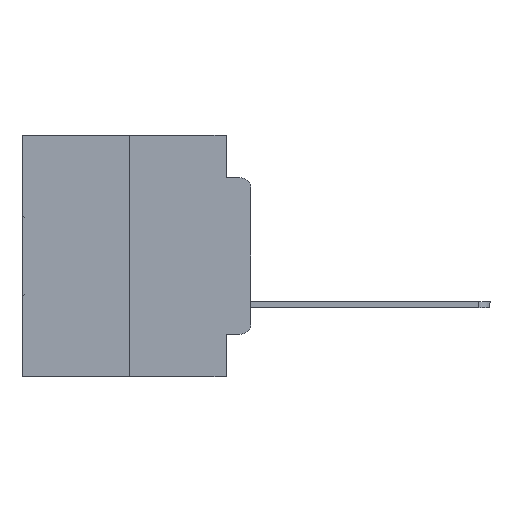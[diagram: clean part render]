
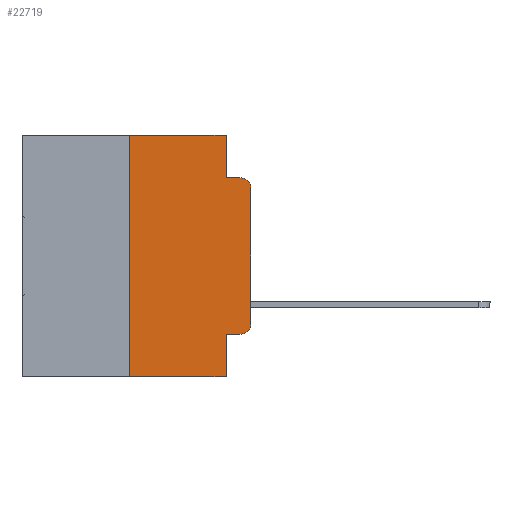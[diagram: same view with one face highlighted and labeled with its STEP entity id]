
A CAD part, left-side view. The second image highlights one B-rep face of the part: STEP entity #22719.
In plain terms, the highlighted planar face has unit normal (-1, 0, 0).
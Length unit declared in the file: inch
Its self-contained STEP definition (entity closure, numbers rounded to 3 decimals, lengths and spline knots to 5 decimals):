
#264 = DIRECTION ( 'NONE',  ( 0., -1., 0. ) ) ;
#451 = EDGE_CURVE ( 'NONE', #6566, #6896, #15571, .T. ) ;
#666 = VERTEX_POINT ( 'NONE', #14685 ) ;
#724 = EDGE_CURVE ( 'NONE', #666, #9016, #13957, .T. ) ;
#1267 = ORIENTED_EDGE ( 'NONE', *, *, #21734, .F. ) ;
#2016 = EDGE_CURVE ( 'NONE', #6903, #4729, #30139, .T. ) ;
#2399 = CARTESIAN_POINT ( 'NONE',  ( 0., 0.051, -0.4115 ) ) ;
#2629 = CARTESIAN_POINT ( 'NONE',  ( 0., 0.051, -0.0885 ) ) ;
#4120 = VECTOR ( 'NONE', #4878, 39.37008 ) ;
#4317 = ORIENTED_EDGE ( 'NONE', *, *, #24093, .F. ) ;
#4729 = VERTEX_POINT ( 'NONE', #5276 ) ;
#4870 = CARTESIAN_POINT ( 'NONE',  ( 0., 0.051, -0.0885 ) ) ;
#4878 = DIRECTION ( 'NONE',  ( 0., 0., 1. ) ) ;
#5249 = AXIS2_PLACEMENT_3D ( 'NONE', #32288, #24366, #12070 ) ;
#5276 = CARTESIAN_POINT ( 'NONE',  ( 0., 0.051, -0.5 ) ) ;
#5303 = ORIENTED_EDGE ( 'NONE', *, *, #2016, .F. ) ;
#6208 = CARTESIAN_POINT ( 'NONE',  ( 0., 0.051, 0. ) ) ;
#6566 = VERTEX_POINT ( 'NONE', #25205 ) ;
#6845 = CIRCLE ( 'NONE', #5249, 0.02 ) ;
#6870 = EDGE_CURVE ( 'NONE', #9016, #17054, #7037, .T. ) ;
#6896 = VERTEX_POINT ( 'NONE', #24810 ) ;
#6903 = VERTEX_POINT ( 'NONE', #29926 ) ;
#7037 = LINE ( 'NONE', #27613, #4120 ) ;
#7404 = DIRECTION ( 'NONE',  ( 0., 0., -1. ) ) ;
#8459 = EDGE_CURVE ( 'NONE', #6903, #666, #19506, .T. ) ;
#8486 = VECTOR ( 'NONE', #30103, 39.37008 ) ;
#9016 = VERTEX_POINT ( 'NONE', #17966 ) ;
#9528 = CARTESIAN_POINT ( 'NONE',  ( 0., 0.02, -0.3915 ) ) ;
#9905 = ORIENTED_EDGE ( 'NONE', *, *, #724, .T. ) ;
#10601 = CARTESIAN_POINT ( 'NONE',  ( 0., 0.25, 0. ) ) ;
#11735 = DIRECTION ( 'NONE',  ( 0., 0., -1. ) ) ;
#12070 = DIRECTION ( 'NONE',  ( 0., 0., -1. ) ) ;
#12193 = DIRECTION ( 'NONE',  ( -1., 0., 0. ) ) ;
#12266 = DIRECTION ( 'NONE',  ( 0., -1., 0. ) ) ;
#12525 = VECTOR ( 'NONE', #12266, 39.37008 ) ;
#12595 = CARTESIAN_POINT ( 'NONE',  ( 0., 0., -0.1085 ) ) ;
#13957 = CIRCLE ( 'NONE', #17136, 0.02 ) ;
#14685 = CARTESIAN_POINT ( 'NONE',  ( 0., 0.02, -0.4115 ) ) ;
#15571 = LINE ( 'NONE', #10601, #27659 ) ;
#15841 = DIRECTION ( 'NONE',  ( 0., -1., 0. ) ) ;
#16435 = VERTEX_POINT ( 'NONE', #28779 ) ;
#17054 = VERTEX_POINT ( 'NONE', #12595 ) ;
#17136 = AXIS2_PLACEMENT_3D ( 'NONE', #9528, #12193, #22322 ) ;
#17444 = ORIENTED_EDGE ( 'NONE', *, *, #6870, .T. ) ;
#17519 = EDGE_CURVE ( 'NONE', #6896, #16435, #20186, .T. ) ;
#17909 = DIRECTION ( 'NONE',  ( 0., 0., 1. ) ) ;
#17966 = CARTESIAN_POINT ( 'NONE',  ( 0., 0., -0.3915 ) ) ;
#18014 = CARTESIAN_POINT ( 'NONE',  ( 0., 0.473, -0.5 ) ) ;
#18182 = CARTESIAN_POINT ( 'NONE',  ( 0., 0.02, -0.0885 ) ) ;
#18297 = AXIS2_PLACEMENT_3D ( 'NONE', #24506, #29794, #7404 ) ;
#18339 = LINE ( 'NONE', #18014, #28554 ) ;
#18352 = DIRECTION ( 'NONE',  ( 0., 0., -1. ) ) ;
#18648 = EDGE_CURVE ( 'NONE', #17054, #21561, #6845, .T. ) ;
#18996 = LINE ( 'NONE', #6208, #30937 ) ;
#19506 = LINE ( 'NONE', #2399, #8486 ) ;
#19689 = FACE_OUTER_BOUND ( 'NONE', #26710, .T. ) ;
#19736 = LINE ( 'NONE', #2629, #12525 ) ;
#20086 = VECTOR ( 'NONE', #11735, 39.37008 ) ;
#20186 = LINE ( 'NONE', #29801, #31661 ) ;
#21536 = ORIENTED_EDGE ( 'NONE', *, *, #28408, .T. ) ;
#21561 = VERTEX_POINT ( 'NONE', #18182 ) ;
#21734 = EDGE_CURVE ( 'NONE', #16435, #22006, #18996, .T. ) ;
#22006 = VERTEX_POINT ( 'NONE', #4870 ) ;
#22322 = DIRECTION ( 'NONE',  ( 0., 0., -1. ) ) ;
#22719 = ADVANCED_FACE ( 'NONE', ( #19689 ), #32107, .F. ) ;
#24093 = EDGE_CURVE ( 'NONE', #22006, #21561, #19736, .T. ) ;
#24267 = ORIENTED_EDGE ( 'NONE', *, *, #18648, .T. ) ;
#24366 = DIRECTION ( 'NONE',  ( -1., 0., 0. ) ) ;
#24506 = CARTESIAN_POINT ( 'NONE',  ( 0., 0.473, 0. ) ) ;
#24518 = CARTESIAN_POINT ( 'NONE',  ( 0., 0.051, 0. ) ) ;
#24810 = CARTESIAN_POINT ( 'NONE',  ( 0., 0.25, 0. ) ) ;
#25205 = CARTESIAN_POINT ( 'NONE',  ( 0., 0.25, -0.5 ) ) ;
#26658 = ORIENTED_EDGE ( 'NONE', *, *, #451, .F. ) ;
#26710 = EDGE_LOOP ( 'NONE', ( #17444, #24267, #4317, #1267, #32604, #26658, #21536, #5303, #30514, #9905 ) ) ;
#27613 = CARTESIAN_POINT ( 'NONE',  ( 0., 0., 0. ) ) ;
#27659 = VECTOR ( 'NONE', #17909, 39.37008 ) ;
#28408 = EDGE_CURVE ( 'NONE', #6566, #4729, #18339, .T. ) ;
#28554 = VECTOR ( 'NONE', #15841, 39.37008 ) ;
#28779 = CARTESIAN_POINT ( 'NONE',  ( 0., 0.051, 0. ) ) ;
#29794 = DIRECTION ( 'NONE',  ( 1., 0., 0. ) ) ;
#29801 = CARTESIAN_POINT ( 'NONE',  ( 0., 0.473, 0. ) ) ;
#29926 = CARTESIAN_POINT ( 'NONE',  ( 0., 0.051, -0.4115 ) ) ;
#30103 = DIRECTION ( 'NONE',  ( 0., -1., 0. ) ) ;
#30139 = LINE ( 'NONE', #24518, #20086 ) ;
#30514 = ORIENTED_EDGE ( 'NONE', *, *, #8459, .T. ) ;
#30937 = VECTOR ( 'NONE', #18352, 39.37008 ) ;
#31661 = VECTOR ( 'NONE', #264, 39.37008 ) ;
#32107 = PLANE ( 'NONE',  #18297 ) ;
#32288 = CARTESIAN_POINT ( 'NONE',  ( 0., 0.02, -0.1085 ) ) ;
#32604 = ORIENTED_EDGE ( 'NONE', *, *, #17519, .F. ) ;
